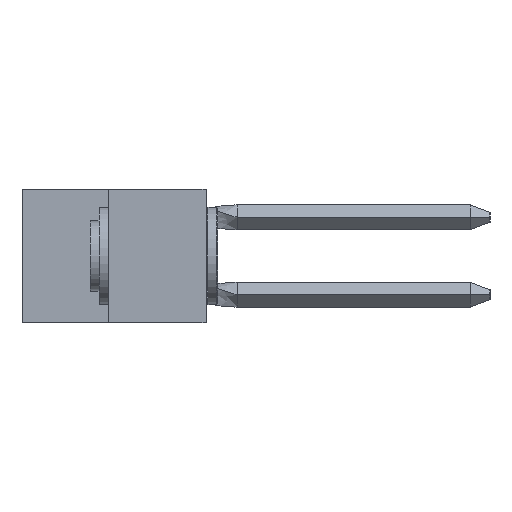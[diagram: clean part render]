
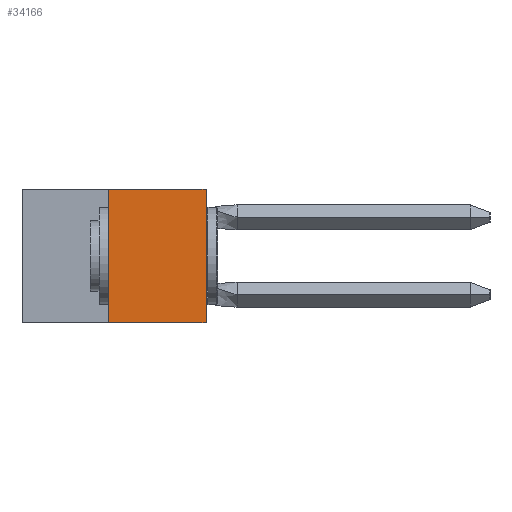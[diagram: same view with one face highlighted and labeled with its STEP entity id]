
A CAD part, left-side view. The second image highlights one B-rep face of the part: STEP entity #34166.
In plain terms, the highlighted planar face has unit normal (-1, 0, 0).
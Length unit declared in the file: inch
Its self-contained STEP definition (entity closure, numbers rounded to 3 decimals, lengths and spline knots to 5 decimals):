
#1194 = ORIENTED_EDGE ( 'NONE', *, *, #39106, .F. ) ;
#1701 = LINE ( 'NONE', #38000, #25082 ) ;
#2759 = EDGE_LOOP ( 'NONE', ( #10156, #1194, #45246, #51596 ) ) ;
#5208 = VERTEX_POINT ( 'NONE', #38971 ) ;
#6182 = EDGE_CURVE ( 'NONE', #38816, #33154, #1701, .T. ) ;
#7436 = CARTESIAN_POINT ( 'NONE',  ( 0., 0.25, -0.343 ) ) ;
#8476 = AXIS2_PLACEMENT_3D ( 'NONE', #17298, #35174, #13231 ) ;
#10156 = ORIENTED_EDGE ( 'NONE', *, *, #16345, .F. ) ;
#13231 = DIRECTION ( 'NONE',  ( 0., 0., -1. ) ) ;
#13903 = CARTESIAN_POINT ( 'NONE',  ( 0., 0.25, 0. ) ) ;
#16345 = EDGE_CURVE ( 'NONE', #5208, #54105, #34798, .T. ) ;
#17298 = CARTESIAN_POINT ( 'NONE',  ( 0., 0.473, 0. ) ) ;
#18348 = DIRECTION ( 'NONE',  ( 0., 0., 1. ) ) ;
#21136 = PLANE ( 'NONE',  #8476 ) ;
#22905 = CARTESIAN_POINT ( 'NONE',  ( 0., 0.473, 0. ) ) ;
#24203 = DIRECTION ( 'NONE',  ( 0., 0., 1. ) ) ;
#25082 = VECTOR ( 'NONE', #56318, 39.37008 ) ;
#29897 = VECTOR ( 'NONE', #18348, 39.37008 ) ;
#31107 = FACE_OUTER_BOUND ( 'NONE', #2759, .T. ) ;
#33154 = VERTEX_POINT ( 'NONE', #40862 ) ;
#33557 = EDGE_CURVE ( 'NONE', #33154, #54105, #56010, .T. ) ;
#34166 = ADVANCED_FACE ( 'NONE', ( #31107 ), #21136, .F. ) ;
#34798 = LINE ( 'NONE', #22905, #40345 ) ;
#35174 = DIRECTION ( 'NONE',  ( 1., 0., 0. ) ) ;
#37275 = CARTESIAN_POINT ( 'NONE',  ( 0., 0., 0. ) ) ;
#38000 = CARTESIAN_POINT ( 'NONE',  ( 0., 0.473, -0.343 ) ) ;
#38816 = VERTEX_POINT ( 'NONE', #7436 ) ;
#38971 = CARTESIAN_POINT ( 'NONE',  ( 0., 0.25, 0. ) ) ;
#39106 = EDGE_CURVE ( 'NONE', #38816, #5208, #56801, .T. ) ;
#40345 = VECTOR ( 'NONE', #53336, 39.37008 ) ;
#40862 = CARTESIAN_POINT ( 'NONE',  ( 0., 0., -0.343 ) ) ;
#42579 = CARTESIAN_POINT ( 'NONE',  ( 0., 0., 0. ) ) ;
#45246 = ORIENTED_EDGE ( 'NONE', *, *, #6182, .T. ) ;
#49808 = VECTOR ( 'NONE', #24203, 39.37008 ) ;
#51596 = ORIENTED_EDGE ( 'NONE', *, *, #33557, .T. ) ;
#53336 = DIRECTION ( 'NONE',  ( 0., -1., 0. ) ) ;
#54105 = VERTEX_POINT ( 'NONE', #42579 ) ;
#56010 = LINE ( 'NONE', #37275, #49808 ) ;
#56318 = DIRECTION ( 'NONE',  ( 0., -1., 0. ) ) ;
#56801 = LINE ( 'NONE', #13903, #29897 ) ;
